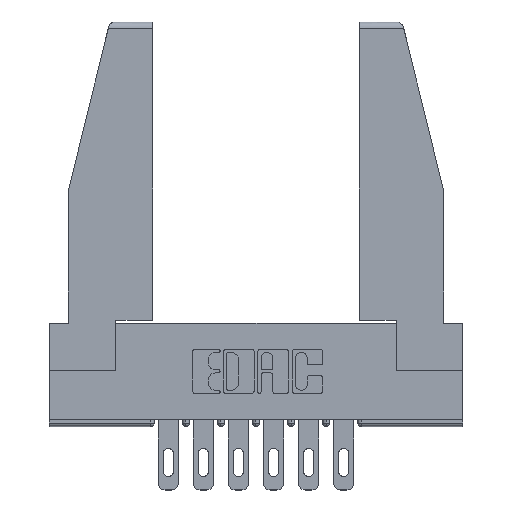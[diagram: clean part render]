
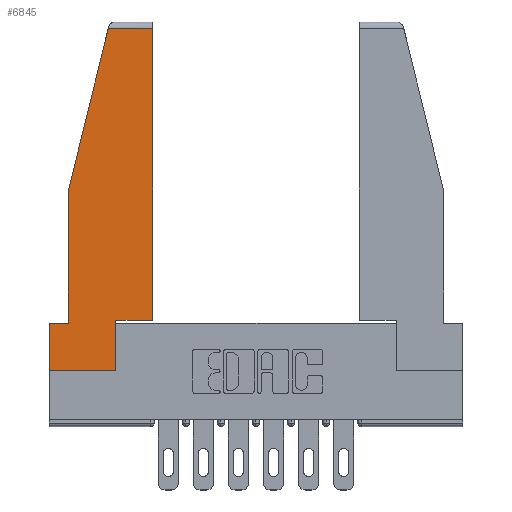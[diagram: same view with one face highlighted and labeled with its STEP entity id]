
A CAD part, top view. The second image highlights one B-rep face of the part: STEP entity #6845.
In plain terms, the highlighted planar face has unit normal (0, 0, 1).
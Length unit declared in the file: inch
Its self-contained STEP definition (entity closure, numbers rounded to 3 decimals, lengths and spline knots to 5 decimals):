
#32 = LINE ( 'NONE', #6472, #7777 ) ;
#67 = VECTOR ( 'NONE', #11628, 39.37008 ) ;
#100 = VERTEX_POINT ( 'NONE', #1832 ) ;
#122 = CARTESIAN_POINT ( 'NONE',  ( 0.461, 1.52, 0. ) ) ;
#340 = VERTEX_POINT ( 'NONE', #4338 ) ;
#396 = VERTEX_POINT ( 'NONE', #10622 ) ;
#565 = EDGE_CURVE ( 'NONE', #10786, #7261, #7136, .T. ) ;
#1023 = EDGE_LOOP ( 'NONE', ( #10383, #7062, #9990, #9408, #13281, #3911, #1510, #2704, #7850 ) ) ;
#1286 = VECTOR ( 'NONE', #11120, 39.37008 ) ;
#1510 = ORIENTED_EDGE ( 'NONE', *, *, #12152, .T. ) ;
#1832 = CARTESIAN_POINT ( 'NONE',  ( 0., 0.21, 0. ) ) ;
#2096 = VECTOR ( 'NONE', #7171, 39.37008 ) ;
#2704 = ORIENTED_EDGE ( 'NONE', *, *, #3989, .T. ) ;
#3335 = CARTESIAN_POINT ( 'NONE',  ( 0.086, 0.21, 0. ) ) ;
#3624 = VERTEX_POINT ( 'NONE', #10535 ) ;
#3711 = CARTESIAN_POINT ( 'NONE',  ( 0.461, 0.223, 0. ) ) ;
#3911 = ORIENTED_EDGE ( 'NONE', *, *, #5384, .T. ) ;
#3959 = DIRECTION ( 'NONE',  ( 0., -1., 0. ) ) ;
#3989 = EDGE_CURVE ( 'NONE', #340, #396, #7427, .T. ) ;
#4020 = CARTESIAN_POINT ( 'NONE',  ( 0.297, 0., 0. ) ) ;
#4338 = CARTESIAN_POINT ( 'NONE',  ( 0.297, 0., 0. ) ) ;
#4742 = FACE_OUTER_BOUND ( 'NONE', #1023, .T. ) ;
#4848 = VERTEX_POINT ( 'NONE', #8725 ) ;
#4967 = VECTOR ( 'NONE', #8300, 39.37008 ) ;
#5095 = CARTESIAN_POINT ( 'NONE',  ( 0.297, 0.223, 0. ) ) ;
#5294 = VERTEX_POINT ( 'NONE', #3335 ) ;
#5384 = EDGE_CURVE ( 'NONE', #100, #12221, #9473, .T. ) ;
#5534 = CARTESIAN_POINT ( 'NONE',  ( 0., 1.52, 0. ) ) ;
#5760 = DIRECTION ( 'NONE',  ( 0., 0., 1. ) ) ;
#6147 = CARTESIAN_POINT ( 'NONE',  ( 0., 0., 0. ) ) ;
#6472 = CARTESIAN_POINT ( 'NONE',  ( 0., 0.21, 0. ) ) ;
#6679 = EDGE_CURVE ( 'NONE', #7261, #3624, #12173, .T. ) ;
#6688 = LINE ( 'NONE', #12683, #11549 ) ;
#6772 = EDGE_CURVE ( 'NONE', #3624, #4848, #6688, .T. ) ;
#6845 = ADVANCED_FACE ( 'NONE', ( #4742 ), #11846, .T. ) ;
#7050 = DIRECTION ( 'NONE',  ( 1., 0., 0. ) ) ;
#7062 = ORIENTED_EDGE ( 'NONE', *, *, #6679, .T. ) ;
#7132 = DIRECTION ( 'NONE',  ( 0., 1., 0. ) ) ;
#7136 = LINE ( 'NONE', #9965, #1286 ) ;
#7171 = DIRECTION ( 'NONE',  ( 1., 0., 0. ) ) ;
#7240 = LINE ( 'NONE', #6147, #4967 ) ;
#7261 = VERTEX_POINT ( 'NONE', #122 ) ;
#7427 = LINE ( 'NONE', #4020, #11948 ) ;
#7434 = CARTESIAN_POINT ( 'NONE',  ( 0., 0., 0. ) ) ;
#7777 = VECTOR ( 'NONE', #10642, 39.37008 ) ;
#7850 = ORIENTED_EDGE ( 'NONE', *, *, #10266, .T. ) ;
#8005 = EDGE_CURVE ( 'NONE', #5294, #100, #32, .T. ) ;
#8300 = DIRECTION ( 'NONE',  ( 1., 0., 0. ) ) ;
#8570 = AXIS2_PLACEMENT_3D ( 'NONE', #11144, #5760, #7050 ) ;
#8578 = LINE ( 'NONE', #5095, #2096 ) ;
#8725 = CARTESIAN_POINT ( 'NONE',  ( 0.086, 0.8, 0. ) ) ;
#8825 = VECTOR ( 'NONE', #12880, 39.37008 ) ;
#9408 = ORIENTED_EDGE ( 'NONE', *, *, #13007, .T. ) ;
#9473 = LINE ( 'NONE', #10630, #8825 ) ;
#9965 = CARTESIAN_POINT ( 'NONE',  ( 0.461, 0.223, 0. ) ) ;
#9990 = ORIENTED_EDGE ( 'NONE', *, *, #6772, .T. ) ;
#10117 = LINE ( 'NONE', #11119, #11590 ) ;
#10266 = EDGE_CURVE ( 'NONE', #396, #10786, #8578, .T. ) ;
#10383 = ORIENTED_EDGE ( 'NONE', *, *, #565, .T. ) ;
#10535 = CARTESIAN_POINT ( 'NONE',  ( 0.2636, 1.52, 0. ) ) ;
#10622 = CARTESIAN_POINT ( 'NONE',  ( 0.297, 0.223, 0. ) ) ;
#10630 = CARTESIAN_POINT ( 'NONE',  ( 0., 0.21, 0. ) ) ;
#10642 = DIRECTION ( 'NONE',  ( -1., 0., 0. ) ) ;
#10786 = VERTEX_POINT ( 'NONE', #3711 ) ;
#11119 = CARTESIAN_POINT ( 'NONE',  ( 0.086, 0.8, 0. ) ) ;
#11120 = DIRECTION ( 'NONE',  ( 0., 1., 0. ) ) ;
#11144 = CARTESIAN_POINT ( 'NONE',  ( 0., 0., 0. ) ) ;
#11182 = DIRECTION ( 'NONE',  ( -0.239, -0.971, 0. ) ) ;
#11549 = VECTOR ( 'NONE', #11182, 39.37008 ) ;
#11590 = VECTOR ( 'NONE', #3959, 39.37008 ) ;
#11628 = DIRECTION ( 'NONE',  ( -1., 0., 0. ) ) ;
#11846 = PLANE ( 'NONE',  #8570 ) ;
#11948 = VECTOR ( 'NONE', #7132, 39.37008 ) ;
#12152 = EDGE_CURVE ( 'NONE', #12221, #340, #7240, .T. ) ;
#12173 = LINE ( 'NONE', #5534, #67 ) ;
#12221 = VERTEX_POINT ( 'NONE', #7434 ) ;
#12683 = CARTESIAN_POINT ( 'NONE',  ( 0.271, 1.55, 0. ) ) ;
#12880 = DIRECTION ( 'NONE',  ( 0., -1., 0. ) ) ;
#13007 = EDGE_CURVE ( 'NONE', #4848, #5294, #10117, .T. ) ;
#13281 = ORIENTED_EDGE ( 'NONE', *, *, #8005, .T. ) ;
